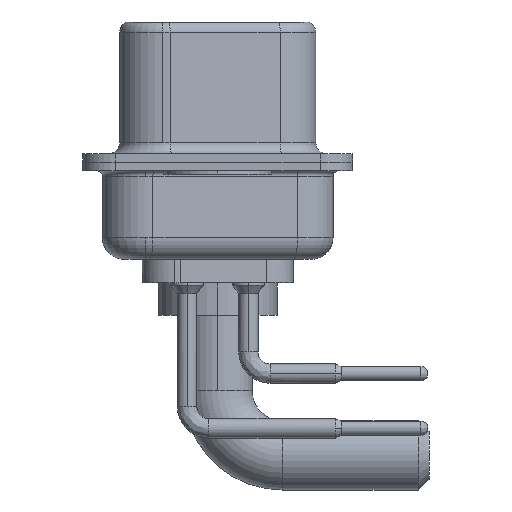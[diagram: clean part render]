
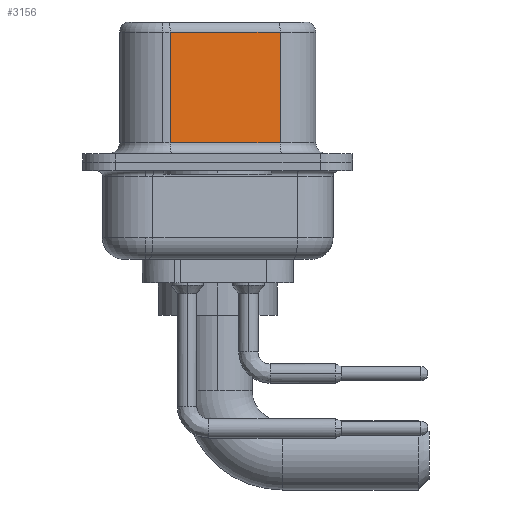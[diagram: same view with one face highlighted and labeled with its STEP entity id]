
A CAD part, left-side view. The second image highlights one B-rep face of the part: STEP entity #3156.
In plain terms, the highlighted planar face has unit normal (-0.985, -0.174, 0).
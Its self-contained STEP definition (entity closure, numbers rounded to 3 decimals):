
#684 = VECTOR ( 'NONE', #13059, 1000. ) ;
#1288 = DIRECTION ( 'NONE',  ( -0.174, 0.985, 0. ) ) ;
#1708 = CARTESIAN_POINT ( 'NONE',  ( 4.555, -2.897, 6.52 ) ) ;
#1923 = CARTESIAN_POINT ( 'NONE',  ( 4.555, -2.897, 6.02 ) ) ;
#2032 = VECTOR ( 'NONE', #2461, 1000. ) ;
#2263 = ORIENTED_EDGE ( 'NONE', *, *, #18108, .T. ) ;
#2292 = AXIS2_PLACEMENT_3D ( 'NONE', #1708, #8064, #1288 ) ;
#2461 = DIRECTION ( 'NONE',  ( 0.174, -0.985, 0. ) ) ;
#2679 = EDGE_LOOP ( 'NONE', ( #19434, #6526, #9077, #2263 ) ) ;
#2682 = VERTEX_POINT ( 'NONE', #3199 ) ;
#3156 = ADVANCED_FACE ( 'NONE', ( #9715 ), #12613, .F. ) ;
#3199 = CARTESIAN_POINT ( 'NONE',  ( 4.555, -2.897, 0.9 ) ) ;
#4500 = EDGE_CURVE ( 'NONE', #19843, #10892, #13449, .T. ) ;
#6526 = ORIENTED_EDGE ( 'NONE', *, *, #4500, .T. ) ;
#6821 = DIRECTION ( 'NONE',  ( -0.174, 0.985, 0. ) ) ;
#8064 = DIRECTION ( 'NONE',  ( 0.985, 0.174, 0. ) ) ;
#8908 = LINE ( 'NONE', #12313, #2032 ) ;
#9077 = ORIENTED_EDGE ( 'NONE', *, *, #11663, .T. ) ;
#9441 = CARTESIAN_POINT ( 'NONE',  ( 4.555, -2.897, 6.52 ) ) ;
#9715 = FACE_OUTER_BOUND ( 'NONE', #2679, .T. ) ;
#10892 = VERTEX_POINT ( 'NONE', #12644 ) ;
#10939 = CARTESIAN_POINT ( 'NONE',  ( 3.655, 2.203, 6.52 ) ) ;
#11095 = LINE ( 'NONE', #9441, #684 ) ;
#11663 = EDGE_CURVE ( 'NONE', #10892, #13560, #14057, .T. ) ;
#11776 = CARTESIAN_POINT ( 'NONE',  ( 4.555, -2.897, 6.02 ) ) ;
#12139 = VECTOR ( 'NONE', #17271, 1000. ) ;
#12313 = CARTESIAN_POINT ( 'NONE',  ( 4.555, -2.897, 0.9 ) ) ;
#12613 = PLANE ( 'NONE',  #2292 ) ;
#12644 = CARTESIAN_POINT ( 'NONE',  ( 3.655, 2.203, 6.02 ) ) ;
#12888 = VECTOR ( 'NONE', #6821, 1000. ) ;
#13059 = DIRECTION ( 'NONE',  ( 0., 0., -1. ) ) ;
#13449 = LINE ( 'NONE', #1923, #12888 ) ;
#13560 = VERTEX_POINT ( 'NONE', #16212 ) ;
#14057 = LINE ( 'NONE', #10939, #12139 ) ;
#16212 = CARTESIAN_POINT ( 'NONE',  ( 3.655, 2.203, 0.9 ) ) ;
#17271 = DIRECTION ( 'NONE',  ( 0., 0., -1. ) ) ;
#17924 = EDGE_CURVE ( 'NONE', #19843, #2682, #11095, .T. ) ;
#18108 = EDGE_CURVE ( 'NONE', #13560, #2682, #8908, .T. ) ;
#19434 = ORIENTED_EDGE ( 'NONE', *, *, #17924, .F. ) ;
#19843 = VERTEX_POINT ( 'NONE', #11776 ) ;
